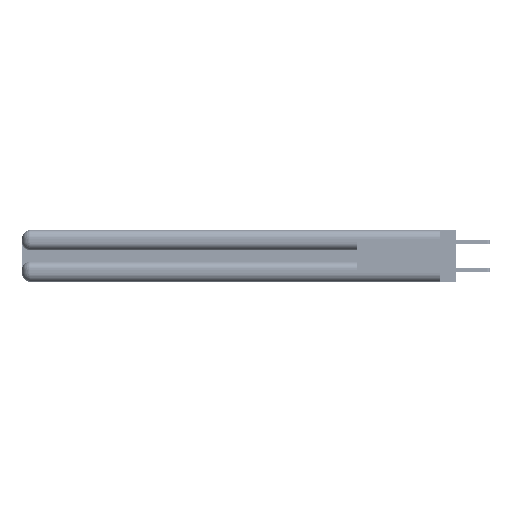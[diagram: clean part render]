
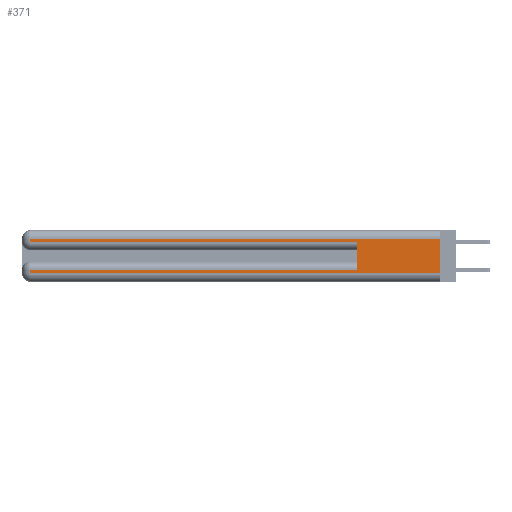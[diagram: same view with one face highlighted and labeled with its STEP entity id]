
A CAD part, left-side view. The second image highlights one B-rep face of the part: STEP entity #371.
In plain terms, the highlighted planar face has unit normal (-1, 0, 0).
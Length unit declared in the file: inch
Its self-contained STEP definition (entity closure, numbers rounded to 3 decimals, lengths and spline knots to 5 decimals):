
#371 = ADVANCED_FACE ( 'NONE', ( #21690 ), #4988, .F. ) ;
#1025 = DIRECTION ( 'NONE',  ( 0., 0., -1. ) ) ;
#1489 = EDGE_CURVE ( 'NONE', #46026, #28265, #45153, .T. ) ;
#2512 = CARTESIAN_POINT ( 'NONE',  ( 0., 0.6, 0.085 ) ) ;
#2816 = VECTOR ( 'NONE', #22554, 39.37008 ) ;
#3353 = DIRECTION ( 'NONE',  ( 0., -1., 0. ) ) ;
#4988 = PLANE ( 'NONE',  #19772 ) ;
#5780 = CARTESIAN_POINT ( 'NONE',  ( 0., 0., 0.06 ) ) ;
#6281 = VERTEX_POINT ( 'NONE', #50319 ) ;
#6634 = EDGE_CURVE ( 'NONE', #18722, #48801, #14265, .T. ) ;
#8779 = DIRECTION ( 'NONE',  ( 1., 0., 0. ) ) ;
#9271 = CARTESIAN_POINT ( 'NONE',  ( 0., 0., 0.085 ) ) ;
#9310 = ORIENTED_EDGE ( 'NONE', *, *, #1489, .T. ) ;
#10221 = CARTESIAN_POINT ( 'NONE',  ( 0., 0., 0.06 ) ) ;
#12294 = EDGE_CURVE ( 'NONE', #39820, #44179, #14586, .T. ) ;
#12837 = VECTOR ( 'NONE', #40892, 39.37008 ) ;
#12919 = VECTOR ( 'NONE', #48805, 39.37008 ) ;
#13133 = ORIENTED_EDGE ( 'NONE', *, *, #12294, .T. ) ;
#13595 = EDGE_CURVE ( 'NONE', #39820, #33663, #25848, .T. ) ;
#14265 = LINE ( 'NONE', #9271, #2816 ) ;
#14416 = VECTOR ( 'NONE', #1025, 39.37008 ) ;
#14586 = LINE ( 'NONE', #28414, #39477 ) ;
#14925 = VECTOR ( 'NONE', #50804, 39.37008 ) ;
#17661 = ORIENTED_EDGE ( 'NONE', *, *, #24215, .F. ) ;
#18722 = VERTEX_POINT ( 'NONE', #2512 ) ;
#19772 = AXIS2_PLACEMENT_3D ( 'NONE', #26594, #8779, #26040 ) ;
#20008 = EDGE_CURVE ( 'NONE', #6281, #33663, #33779, .T. ) ;
#20820 = CARTESIAN_POINT ( 'NONE',  ( 0., 0., 0.285 ) ) ;
#21690 = FACE_OUTER_BOUND ( 'NONE', #35910, .T. ) ;
#22059 = CARTESIAN_POINT ( 'NONE',  ( 0., 0.6, 0.145 ) ) ;
#22554 = DIRECTION ( 'NONE',  ( 0., 1., 0. ) ) ;
#24215 = EDGE_CURVE ( 'NONE', #18722, #28265, #54795, .T. ) ;
#24729 = ORIENTED_EDGE ( 'NONE', *, *, #6634, .T. ) ;
#25675 = ORIENTED_EDGE ( 'NONE', *, *, #20008, .T. ) ;
#25848 = LINE ( 'NONE', #34715, #14416 ) ;
#26040 = DIRECTION ( 'NONE',  ( 0., 0., -1. ) ) ;
#26305 = LINE ( 'NONE', #53157, #12837 ) ;
#26350 = LINE ( 'NONE', #28925, #14925 ) ;
#26594 = CARTESIAN_POINT ( 'NONE',  ( 0., 0., 0.37 ) ) ;
#28265 = VERTEX_POINT ( 'NONE', #43168 ) ;
#28414 = CARTESIAN_POINT ( 'NONE',  ( 0., 0., 0.31 ) ) ;
#28925 = CARTESIAN_POINT ( 'NONE',  ( 0., 2.94, 0.37 ) ) ;
#29259 = EDGE_CURVE ( 'NONE', #44179, #46026, #26350, .T. ) ;
#30548 = DIRECTION ( 'NONE',  ( 0., 0., 1. ) ) ;
#32526 = ORIENTED_EDGE ( 'NONE', *, *, #29259, .T. ) ;
#32559 = VECTOR ( 'NONE', #30548, 39.37008 ) ;
#33663 = VERTEX_POINT ( 'NONE', #5780 ) ;
#33779 = LINE ( 'NONE', #10221, #12919 ) ;
#34715 = CARTESIAN_POINT ( 'NONE',  ( 0., 0., 0.37 ) ) ;
#35910 = EDGE_LOOP ( 'NONE', ( #45512, #13133, #32526, #9310, #17661, #24729, #52493, #25675 ) ) ;
#37008 = CARTESIAN_POINT ( 'NONE',  ( 0., 2.94, 0.285 ) ) ;
#39477 = VECTOR ( 'NONE', #45573, 39.37008 ) ;
#39820 = VERTEX_POINT ( 'NONE', #41586 ) ;
#40842 = CARTESIAN_POINT ( 'NONE',  ( 0., 2.94, 0.085 ) ) ;
#40892 = DIRECTION ( 'NONE',  ( 0., 0., -1. ) ) ;
#41586 = CARTESIAN_POINT ( 'NONE',  ( 0., 0., 0.31 ) ) ;
#42432 = VECTOR ( 'NONE', #3353, 39.37008 ) ;
#43168 = CARTESIAN_POINT ( 'NONE',  ( 0., 0.6, 0.285 ) ) ;
#44179 = VERTEX_POINT ( 'NONE', #52588 ) ;
#45153 = LINE ( 'NONE', #20820, #42432 ) ;
#45512 = ORIENTED_EDGE ( 'NONE', *, *, #13595, .F. ) ;
#45573 = DIRECTION ( 'NONE',  ( 0., 1., 0. ) ) ;
#46026 = VERTEX_POINT ( 'NONE', #37008 ) ;
#48801 = VERTEX_POINT ( 'NONE', #40842 ) ;
#48805 = DIRECTION ( 'NONE',  ( 0., -1., 0. ) ) ;
#50100 = EDGE_CURVE ( 'NONE', #48801, #6281, #26305, .T. ) ;
#50319 = CARTESIAN_POINT ( 'NONE',  ( 0., 2.94, 0.06 ) ) ;
#50804 = DIRECTION ( 'NONE',  ( 0., 0., -1. ) ) ;
#52493 = ORIENTED_EDGE ( 'NONE', *, *, #50100, .T. ) ;
#52588 = CARTESIAN_POINT ( 'NONE',  ( 0., 2.94, 0.31 ) ) ;
#53157 = CARTESIAN_POINT ( 'NONE',  ( 0., 2.94, 0.37 ) ) ;
#54795 = LINE ( 'NONE', #22059, #32559 ) ;
